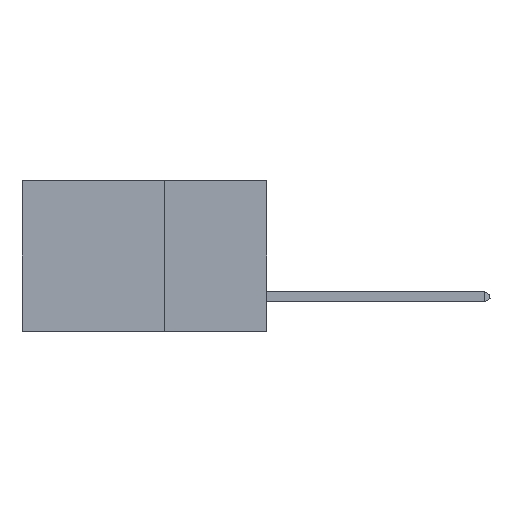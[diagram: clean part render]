
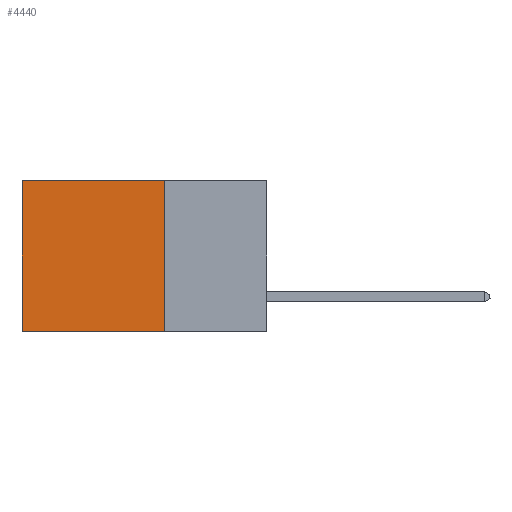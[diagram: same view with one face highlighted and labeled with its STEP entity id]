
A CAD part, left-side view. The second image highlights one B-rep face of the part: STEP entity #4440.
In plain terms, the highlighted planar face has unit normal (-1, 0, 0).
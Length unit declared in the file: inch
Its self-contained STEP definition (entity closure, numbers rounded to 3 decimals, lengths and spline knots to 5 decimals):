
#91 = CARTESIAN_POINT ( 'NONE',  ( 0.2875, 0.25, -0.37 ) ) ;
#331 = VECTOR ( 'NONE', #2771, 39.37008 ) ;
#438 = DIRECTION ( 'NONE',  ( 1., 0., 0. ) ) ;
#1350 = VERTEX_POINT ( 'NONE', #2509 ) ;
#1982 = VERTEX_POINT ( 'NONE', #3868 ) ;
#2161 = CARTESIAN_POINT ( 'NONE',  ( 0.2875, 0.6, -0.37 ) ) ;
#2509 = CARTESIAN_POINT ( 'NONE',  ( 0.2875, 0.25, 0. ) ) ;
#2543 = EDGE_CURVE ( 'NONE', #1350, #2770, #7915, .T. ) ;
#2770 = VERTEX_POINT ( 'NONE', #91 ) ;
#2771 = DIRECTION ( 'NONE',  ( 0., 0., -1. ) ) ;
#3499 = DIRECTION ( 'NONE',  ( 0., 1., 0. ) ) ;
#3624 = LINE ( 'NONE', #13719, #11309 ) ;
#3868 = CARTESIAN_POINT ( 'NONE',  ( 0.2875, 0.6, 0. ) ) ;
#3918 = AXIS2_PLACEMENT_3D ( 'NONE', #7356, #438, #5032 ) ;
#3977 = EDGE_CURVE ( 'NONE', #1982, #9471, #13095, .T. ) ;
#4440 = ADVANCED_FACE ( 'NONE', ( #12156 ), #11806, .F. ) ;
#4709 = CARTESIAN_POINT ( 'NONE',  ( 0.2875, 0.25, 0. ) ) ;
#4807 = EDGE_CURVE ( 'NONE', #1350, #1982, #14482, .T. ) ;
#5032 = DIRECTION ( 'NONE',  ( 0., 0., -1. ) ) ;
#6149 = DIRECTION ( 'NONE',  ( 0., 0., -1. ) ) ;
#6700 = ORIENTED_EDGE ( 'NONE', *, *, #4807, .T. ) ;
#7223 = CARTESIAN_POINT ( 'NONE',  ( 0.2875, 0.6, 0. ) ) ;
#7356 = CARTESIAN_POINT ( 'NONE',  ( 0.2875, 0.25, 0. ) ) ;
#7887 = DIRECTION ( 'NONE',  ( 0., 1., 0. ) ) ;
#7913 = CARTESIAN_POINT ( 'NONE',  ( 0.2875, 0.25, 0. ) ) ;
#7915 = LINE ( 'NONE', #7913, #11129 ) ;
#8836 = ORIENTED_EDGE ( 'NONE', *, *, #2543, .F. ) ;
#9159 = ORIENTED_EDGE ( 'NONE', *, *, #3977, .T. ) ;
#9194 = EDGE_LOOP ( 'NONE', ( #9159, #9329, #8836, #6700 ) ) ;
#9329 = ORIENTED_EDGE ( 'NONE', *, *, #11751, .F. ) ;
#9471 = VERTEX_POINT ( 'NONE', #2161 ) ;
#11129 = VECTOR ( 'NONE', #6149, 39.37008 ) ;
#11309 = VECTOR ( 'NONE', #7887, 39.37008 ) ;
#11751 = EDGE_CURVE ( 'NONE', #2770, #9471, #3624, .T. ) ;
#11806 = PLANE ( 'NONE',  #3918 ) ;
#12156 = FACE_OUTER_BOUND ( 'NONE', #9194, .T. ) ;
#13095 = LINE ( 'NONE', #7223, #331 ) ;
#13241 = VECTOR ( 'NONE', #3499, 39.37008 ) ;
#13719 = CARTESIAN_POINT ( 'NONE',  ( 0.2875, 0.25, -0.37 ) ) ;
#14482 = LINE ( 'NONE', #4709, #13241 ) ;
